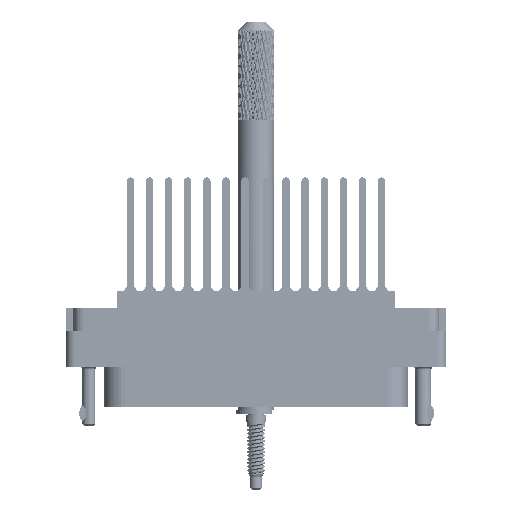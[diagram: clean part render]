
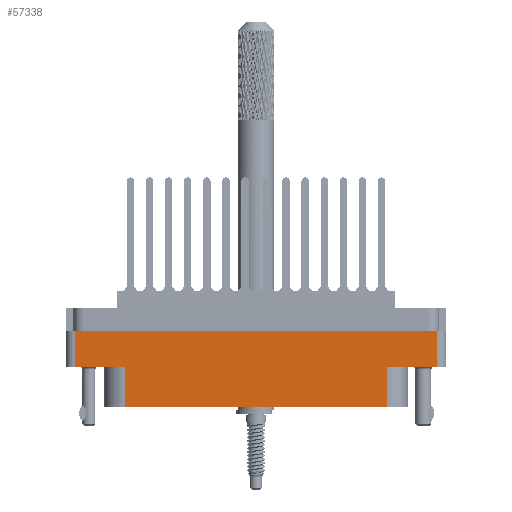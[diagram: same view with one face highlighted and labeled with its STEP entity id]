
A CAD part, front view. The second image highlights one B-rep face of the part: STEP entity #57338.
In plain terms, the highlighted planar face has unit normal (0, -1, 0).
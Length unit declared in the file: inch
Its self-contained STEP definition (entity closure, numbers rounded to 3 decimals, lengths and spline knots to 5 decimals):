
#130 = ORIENTED_EDGE ( 'NONE', *, *, #94954, .F. ) ;
#749 = VERTEX_POINT ( 'NONE', #54239 ) ;
#1307 = DIRECTION ( 'NONE',  ( 0., 0., -1. ) ) ;
#1773 = VERTEX_POINT ( 'NONE', #70735 ) ;
#1841 = FACE_OUTER_BOUND ( 'NONE', #97567, .T. ) ;
#9300 = EDGE_CURVE ( 'NONE', #65461, #749, #27161, .T. ) ;
#14029 = LINE ( 'NONE', #61669, #122190 ) ;
#14577 = LINE ( 'NONE', #115511, #74789 ) ;
#20942 = EDGE_CURVE ( 'NONE', #23702, #101792, #111845, .T. ) ;
#23702 = VERTEX_POINT ( 'NONE', #85946 ) ;
#27161 = LINE ( 'NONE', #108066, #66283 ) ;
#30065 = CARTESIAN_POINT ( 'NONE',  ( 0.895, -0.438, -0.789 ) ) ;
#33489 = ORIENTED_EDGE ( 'NONE', *, *, #9300, .F. ) ;
#36401 = VECTOR ( 'NONE', #45401, 39.37008 ) ;
#38192 = VECTOR ( 'NONE', #118179, 39.37008 ) ;
#38263 = VECTOR ( 'NONE', #108404, 39.37008 ) ;
#40079 = DIRECTION ( 'NONE',  ( 1., 0., 0. ) ) ;
#45401 = DIRECTION ( 'NONE',  ( -1., 0., 0. ) ) ;
#47283 = VECTOR ( 'NONE', #76702, 39.37008 ) ;
#51463 = LINE ( 'NONE', #65189, #36401 ) ;
#54239 = CARTESIAN_POINT ( 'NONE',  ( 0.895, -0.438, -0.52 ) ) ;
#54678 = LINE ( 'NONE', #90561, #38192 ) ;
#54723 = ORIENTED_EDGE ( 'NONE', *, *, #20942, .T. ) ;
#57338 = ADVANCED_FACE ( 'NONE', ( #1841 ), #106066, .T. ) ;
#58617 = CARTESIAN_POINT ( 'NONE',  ( 0., -0.438, -0.274 ) ) ;
#60593 = CARTESIAN_POINT ( 'NONE',  ( -1.2335, -0.438, -0.52 ) ) ;
#61669 = CARTESIAN_POINT ( 'NONE',  ( 1.2335, -0.438, -0.789 ) ) ;
#63301 = ORIENTED_EDGE ( 'NONE', *, *, #94388, .T. ) ;
#63734 = VERTEX_POINT ( 'NONE', #60593 ) ;
#64722 = EDGE_CURVE ( 'NONE', #1773, #63734, #14577, .T. ) ;
#65189 = CARTESIAN_POINT ( 'NONE',  ( 0., -0.438, -0.52 ) ) ;
#65461 = VERTEX_POINT ( 'NONE', #111861 ) ;
#66283 = VECTOR ( 'NONE', #80844, 39.37008 ) ;
#67523 = CARTESIAN_POINT ( 'NONE',  ( -1.2955, -0.438, -0.789 ) ) ;
#69035 = CARTESIAN_POINT ( 'NONE',  ( -0.895, -0.438, -0.789 ) ) ;
#70735 = CARTESIAN_POINT ( 'NONE',  ( -1.2335, -0.438, -0.274 ) ) ;
#74674 = ORIENTED_EDGE ( 'NONE', *, *, #88735, .T. ) ;
#74789 = VECTOR ( 'NONE', #1307, 39.37008 ) ;
#76702 = DIRECTION ( 'NONE',  ( 1., 0., 0. ) ) ;
#77285 = CARTESIAN_POINT ( 'NONE',  ( 1.2335, -0.438, -0.274 ) ) ;
#78584 = ORIENTED_EDGE ( 'NONE', *, *, #64722, .T. ) ;
#80844 = DIRECTION ( 'NONE',  ( -1., 0., 0. ) ) ;
#81854 = DIRECTION ( 'NONE',  ( 0., 0., 1. ) ) ;
#82077 = VERTEX_POINT ( 'NONE', #77285 ) ;
#85946 = CARTESIAN_POINT ( 'NONE',  ( -0.895, -0.438, -0.52 ) ) ;
#86495 = ORIENTED_EDGE ( 'NONE', *, *, #114660, .F. ) ;
#86746 = VECTOR ( 'NONE', #40079, 39.37008 ) ;
#88576 = VERTEX_POINT ( 'NONE', #30065 ) ;
#88735 = EDGE_CURVE ( 'NONE', #88576, #749, #54678, .T. ) ;
#90561 = CARTESIAN_POINT ( 'NONE',  ( 0.895, -0.438, -0.52 ) ) ;
#90898 = AXIS2_PLACEMENT_3D ( 'NONE', #67523, #104405, #123699 ) ;
#94388 = EDGE_CURVE ( 'NONE', #65461, #82077, #14029, .T. ) ;
#94954 = EDGE_CURVE ( 'NONE', #23702, #63734, #51463, .T. ) ;
#95447 = ORIENTED_EDGE ( 'NONE', *, *, #109499, .T. ) ;
#97567 = EDGE_LOOP ( 'NONE', ( #86495, #78584, #130, #54723, #95447, #74674, #33489, #63301 ) ) ;
#101792 = VERTEX_POINT ( 'NONE', #110250 ) ;
#104405 = DIRECTION ( 'NONE',  ( 0., -1., 0. ) ) ;
#105851 = LINE ( 'NONE', #122820, #47283 ) ;
#106066 = PLANE ( 'NONE',  #90898 ) ;
#108066 = CARTESIAN_POINT ( 'NONE',  ( 0., -0.438, -0.52 ) ) ;
#108404 = DIRECTION ( 'NONE',  ( 0., 0., -1. ) ) ;
#109499 = EDGE_CURVE ( 'NONE', #101792, #88576, #105851, .T. ) ;
#110250 = CARTESIAN_POINT ( 'NONE',  ( -0.895, -0.438, -0.789 ) ) ;
#111845 = LINE ( 'NONE', #69035, #38263 ) ;
#111861 = CARTESIAN_POINT ( 'NONE',  ( 1.2335, -0.438, -0.52 ) ) ;
#112111 = LINE ( 'NONE', #58617, #86746 ) ;
#114660 = EDGE_CURVE ( 'NONE', #1773, #82077, #112111, .T. ) ;
#115511 = CARTESIAN_POINT ( 'NONE',  ( -1.2335, -0.438, -0.789 ) ) ;
#118179 = DIRECTION ( 'NONE',  ( 0., 0., 1. ) ) ;
#122190 = VECTOR ( 'NONE', #81854, 39.37008 ) ;
#122820 = CARTESIAN_POINT ( 'NONE',  ( -1.2955, -0.438, -0.789 ) ) ;
#123699 = DIRECTION ( 'NONE',  ( 0., 0., -1. ) ) ;
